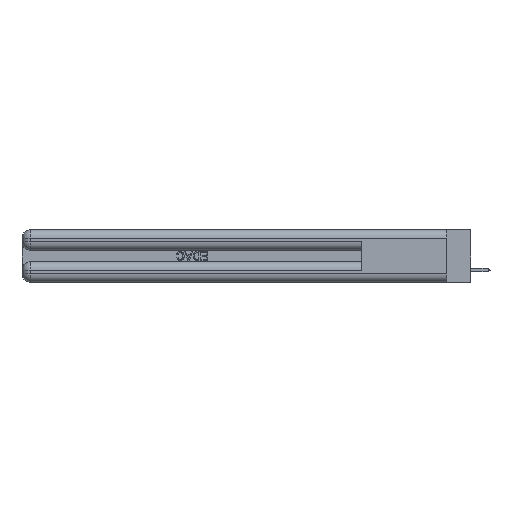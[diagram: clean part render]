
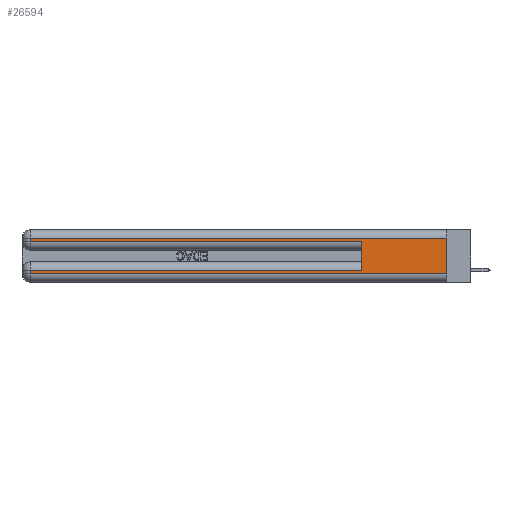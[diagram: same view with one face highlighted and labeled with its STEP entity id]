
A CAD part, left-side view. The second image highlights one B-rep face of the part: STEP entity #26594.
In plain terms, the highlighted planar face has unit normal (-1, 0, 0).
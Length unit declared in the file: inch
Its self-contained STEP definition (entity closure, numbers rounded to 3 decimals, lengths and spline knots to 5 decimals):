
#30 = VECTOR ( 'NONE', #24705, 39.37008 ) ;
#118 = DIRECTION ( 'NONE',  ( 1., 0., 0. ) ) ;
#648 = LINE ( 'NONE', #2481, #29110 ) ;
#707 = VERTEX_POINT ( 'NONE', #18109 ) ;
#956 = VECTOR ( 'NONE', #10974, 39.37008 ) ;
#1078 = VERTEX_POINT ( 'NONE', #9247 ) ;
#1386 = DIRECTION ( 'NONE',  ( 0., 1., 0. ) ) ;
#2481 = CARTESIAN_POINT ( 'NONE',  ( 0., 2.94, 0.37 ) ) ;
#3130 = PLANE ( 'NONE',  #39977 ) ;
#6253 = EDGE_LOOP ( 'NONE', ( #18498, #38900, #37181, #13849, #7488, #30750, #26211, #41378 ) ) ;
#6848 = CARTESIAN_POINT ( 'NONE',  ( 0., 2.94, 0.06 ) ) ;
#7441 = DIRECTION ( 'NONE',  ( 0., 0., 1. ) ) ;
#7488 = ORIENTED_EDGE ( 'NONE', *, *, #39845, .F. ) ;
#7514 = LINE ( 'NONE', #24429, #15034 ) ;
#8099 = CARTESIAN_POINT ( 'NONE',  ( 0., 0., 0.085 ) ) ;
#9080 = DIRECTION ( 'NONE',  ( 0., 0., -1. ) ) ;
#9221 = LINE ( 'NONE', #32572, #25947 ) ;
#9247 = CARTESIAN_POINT ( 'NONE',  ( 0., 0.6, 0.285 ) ) ;
#9795 = VERTEX_POINT ( 'NONE', #12193 ) ;
#10384 = DIRECTION ( 'NONE',  ( 0., 1., 0. ) ) ;
#10550 = VECTOR ( 'NONE', #10384, 39.37008 ) ;
#10974 = DIRECTION ( 'NONE',  ( 0., 0., -1. ) ) ;
#12193 = CARTESIAN_POINT ( 'NONE',  ( 0., 0., 0.31 ) ) ;
#12259 = DIRECTION ( 'NONE',  ( 0., -1., 0. ) ) ;
#13097 = VECTOR ( 'NONE', #17387, 39.37008 ) ;
#13849 = ORIENTED_EDGE ( 'NONE', *, *, #25303, .T. ) ;
#14369 = EDGE_CURVE ( 'NONE', #19762, #30022, #648, .T. ) ;
#14731 = CARTESIAN_POINT ( 'NONE',  ( 0., 0., 0.06 ) ) ;
#15034 = VECTOR ( 'NONE', #7441, 39.37008 ) ;
#16830 = VERTEX_POINT ( 'NONE', #14731 ) ;
#17387 = DIRECTION ( 'NONE',  ( 0., -1., 0. ) ) ;
#18109 = CARTESIAN_POINT ( 'NONE',  ( 0., 2.94, 0.285 ) ) ;
#18430 = CARTESIAN_POINT ( 'NONE',  ( 0., 2.94, 0.31 ) ) ;
#18498 = ORIENTED_EDGE ( 'NONE', *, *, #40104, .F. ) ;
#19762 = VERTEX_POINT ( 'NONE', #38974 ) ;
#20614 = VECTOR ( 'NONE', #1386, 39.37008 ) ;
#21085 = LINE ( 'NONE', #42427, #20614 ) ;
#21723 = FACE_OUTER_BOUND ( 'NONE', #6253, .T. ) ;
#24095 = LINE ( 'NONE', #33902, #956 ) ;
#24162 = CARTESIAN_POINT ( 'NONE',  ( 0., 0., 0.285 ) ) ;
#24429 = CARTESIAN_POINT ( 'NONE',  ( 0., 0.6, 0.145 ) ) ;
#24705 = DIRECTION ( 'NONE',  ( 0., 0., -1. ) ) ;
#25303 = EDGE_CURVE ( 'NONE', #707, #1078, #31764, .T. ) ;
#25781 = CARTESIAN_POINT ( 'NONE',  ( 0., 0., 0.37 ) ) ;
#25947 = VECTOR ( 'NONE', #12259, 39.37008 ) ;
#26211 = ORIENTED_EDGE ( 'NONE', *, *, #14369, .T. ) ;
#26594 = ADVANCED_FACE ( 'NONE', ( #21723 ), #3130, .F. ) ;
#27871 = LINE ( 'NONE', #25781, #30 ) ;
#29110 = VECTOR ( 'NONE', #9080, 39.37008 ) ;
#29691 = VERTEX_POINT ( 'NONE', #18430 ) ;
#30022 = VERTEX_POINT ( 'NONE', #6848 ) ;
#30277 = CARTESIAN_POINT ( 'NONE',  ( 0., 0.6, 0.085 ) ) ;
#30750 = ORIENTED_EDGE ( 'NONE', *, *, #42518, .T. ) ;
#31764 = LINE ( 'NONE', #24162, #13097 ) ;
#32572 = CARTESIAN_POINT ( 'NONE',  ( 0., 0., 0.06 ) ) ;
#33716 = EDGE_CURVE ( 'NONE', #9795, #29691, #21085, .T. ) ;
#33902 = CARTESIAN_POINT ( 'NONE',  ( 0., 2.94, 0.37 ) ) ;
#34548 = DIRECTION ( 'NONE',  ( 0., 0., -1. ) ) ;
#34777 = EDGE_CURVE ( 'NONE', #30022, #16830, #9221, .T. ) ;
#37181 = ORIENTED_EDGE ( 'NONE', *, *, #40663, .T. ) ;
#37872 = LINE ( 'NONE', #8099, #10550 ) ;
#38900 = ORIENTED_EDGE ( 'NONE', *, *, #33716, .T. ) ;
#38974 = CARTESIAN_POINT ( 'NONE',  ( 0., 2.94, 0.085 ) ) ;
#39845 = EDGE_CURVE ( 'NONE', #44148, #1078, #7514, .T. ) ;
#39977 = AXIS2_PLACEMENT_3D ( 'NONE', #44280, #118, #34548 ) ;
#40104 = EDGE_CURVE ( 'NONE', #9795, #16830, #27871, .T. ) ;
#40663 = EDGE_CURVE ( 'NONE', #29691, #707, #24095, .T. ) ;
#41378 = ORIENTED_EDGE ( 'NONE', *, *, #34777, .T. ) ;
#42427 = CARTESIAN_POINT ( 'NONE',  ( 0., 0., 0.31 ) ) ;
#42518 = EDGE_CURVE ( 'NONE', #44148, #19762, #37872, .T. ) ;
#44148 = VERTEX_POINT ( 'NONE', #30277 ) ;
#44280 = CARTESIAN_POINT ( 'NONE',  ( 0., 0., 0.37 ) ) ;
